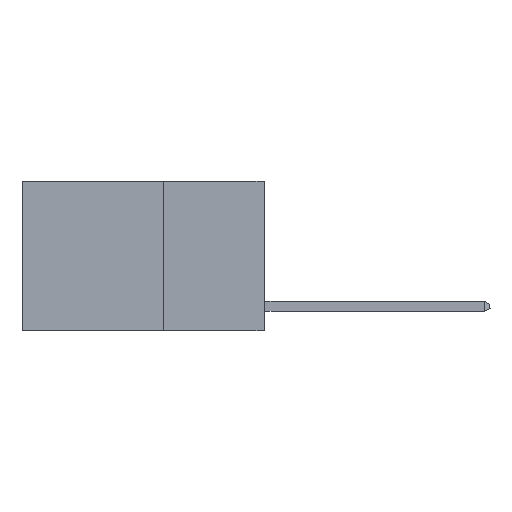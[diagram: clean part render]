
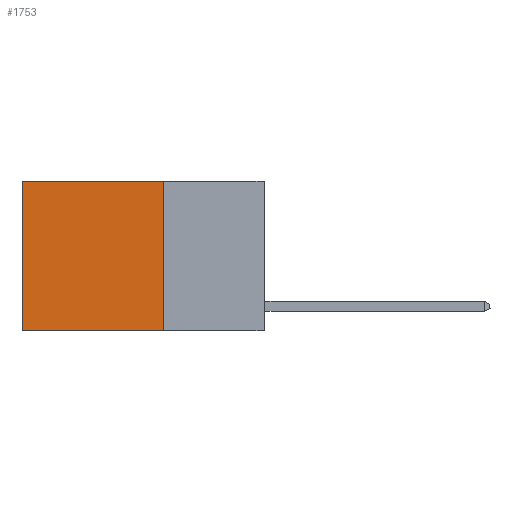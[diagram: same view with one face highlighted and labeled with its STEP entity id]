
A CAD part, left-side view. The second image highlights one B-rep face of the part: STEP entity #1753.
In plain terms, the highlighted planar face has unit normal (-1, 0, 0).
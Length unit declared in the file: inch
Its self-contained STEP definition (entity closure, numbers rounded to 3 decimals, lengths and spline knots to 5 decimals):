
#172 = DIRECTION ( 'NONE',  ( 0., 0., -1. ) ) ;
#458 = LINE ( 'NONE', #10224, #11829 ) ;
#1292 = CARTESIAN_POINT ( 'NONE',  ( 0.2625, 0.6, -0.37 ) ) ;
#1753 = ADVANCED_FACE ( 'NONE', ( #12434 ), #10861, .F. ) ;
#2208 = CARTESIAN_POINT ( 'NONE',  ( 0.2625, 0.25, -0.37 ) ) ;
#2392 = ORIENTED_EDGE ( 'NONE', *, *, #20938, .T. ) ;
#2931 = AXIS2_PLACEMENT_3D ( 'NONE', #26572, #28837, #15373 ) ;
#3198 = LINE ( 'NONE', #13833, #20490 ) ;
#4932 = VERTEX_POINT ( 'NONE', #29047 ) ;
#6200 = VERTEX_POINT ( 'NONE', #2208 ) ;
#8527 = ORIENTED_EDGE ( 'NONE', *, *, #21446, .F. ) ;
#9047 = CARTESIAN_POINT ( 'NONE',  ( 0.2625, 0.6, 0. ) ) ;
#9916 = VERTEX_POINT ( 'NONE', #1292 ) ;
#10224 = CARTESIAN_POINT ( 'NONE',  ( 0.2625, 0.25, 0. ) ) ;
#10258 = EDGE_CURVE ( 'NONE', #4932, #6200, #19479, .T. ) ;
#10861 = PLANE ( 'NONE',  #2931 ) ;
#11829 = VECTOR ( 'NONE', #12471, 39.37008 ) ;
#12434 = FACE_OUTER_BOUND ( 'NONE', #14724, .T. ) ;
#12471 = DIRECTION ( 'NONE',  ( 0., 1., 0. ) ) ;
#13833 = CARTESIAN_POINT ( 'NONE',  ( 0.2625, 0.6, 0. ) ) ;
#14201 = VECTOR ( 'NONE', #172, 39.37008 ) ;
#14435 = DIRECTION ( 'NONE',  ( 0., 1., 0. ) ) ;
#14522 = CARTESIAN_POINT ( 'NONE',  ( 0.2625, 0.25, -0.37 ) ) ;
#14724 = EDGE_LOOP ( 'NONE', ( #26471, #8527, #28503, #2392 ) ) ;
#15373 = DIRECTION ( 'NONE',  ( 0., 0., -1. ) ) ;
#16105 = DIRECTION ( 'NONE',  ( 0., 0., -1. ) ) ;
#18639 = VERTEX_POINT ( 'NONE', #9047 ) ;
#19479 = LINE ( 'NONE', #24869, #14201 ) ;
#20490 = VECTOR ( 'NONE', #16105, 39.37008 ) ;
#20938 = EDGE_CURVE ( 'NONE', #4932, #18639, #458, .T. ) ;
#21446 = EDGE_CURVE ( 'NONE', #6200, #9916, #22362, .T. ) ;
#22362 = LINE ( 'NONE', #14522, #27634 ) ;
#23029 = EDGE_CURVE ( 'NONE', #18639, #9916, #3198, .T. ) ;
#24869 = CARTESIAN_POINT ( 'NONE',  ( 0.2625, 0.25, 0. ) ) ;
#26471 = ORIENTED_EDGE ( 'NONE', *, *, #23029, .T. ) ;
#26572 = CARTESIAN_POINT ( 'NONE',  ( 0.2625, 0.25, 0. ) ) ;
#27634 = VECTOR ( 'NONE', #14435, 39.37008 ) ;
#28503 = ORIENTED_EDGE ( 'NONE', *, *, #10258, .F. ) ;
#28837 = DIRECTION ( 'NONE',  ( 1., 0., 0. ) ) ;
#29047 = CARTESIAN_POINT ( 'NONE',  ( 0.2625, 0.25, 0. ) ) ;
